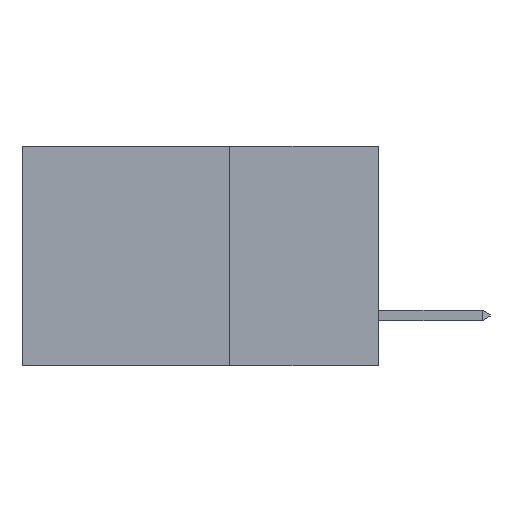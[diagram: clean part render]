
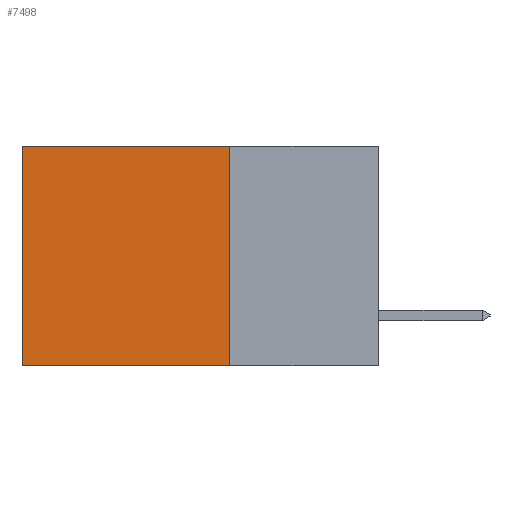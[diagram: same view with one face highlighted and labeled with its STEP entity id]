
A CAD part, left-side view. The second image highlights one B-rep face of the part: STEP entity #7498.
In plain terms, the highlighted planar face has unit normal (-1, 0, 0).
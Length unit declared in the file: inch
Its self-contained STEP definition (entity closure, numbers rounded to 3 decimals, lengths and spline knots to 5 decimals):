
#665 = VECTOR ( 'NONE', #9670, 39.37008 ) ;
#2373 = VERTEX_POINT ( 'NONE', #3122 ) ;
#2735 = VECTOR ( 'NONE', #9588, 39.37008 ) ;
#3122 = CARTESIAN_POINT ( 'NONE',  ( 0.2615, 0.6, 0. ) ) ;
#3633 = CARTESIAN_POINT ( 'NONE',  ( 0.2615, 0.6, -0.37 ) ) ;
#5329 = AXIS2_PLACEMENT_3D ( 'NONE', #10758, #12197, #13166 ) ;
#5588 = ORIENTED_EDGE ( 'NONE', *, *, #11758, .T. ) ;
#5737 = ORIENTED_EDGE ( 'NONE', *, *, #5966, .T. ) ;
#5966 = EDGE_CURVE ( 'NONE', #2373, #10109, #16597, .T. ) ;
#6397 = DIRECTION ( 'NONE',  ( 0., 0., -1. ) ) ;
#6584 = FACE_OUTER_BOUND ( 'NONE', #8172, .T. ) ;
#6719 = ORIENTED_EDGE ( 'NONE', *, *, #12212, .F. ) ;
#6962 = VECTOR ( 'NONE', #8562, 39.37008 ) ;
#7164 = CARTESIAN_POINT ( 'NONE',  ( 0.2615, 0.25, -0.37 ) ) ;
#7402 = LINE ( 'NONE', #7164, #6962 ) ;
#7498 = ADVANCED_FACE ( 'NONE', ( #6584 ), #14477, .F. ) ;
#8172 = EDGE_LOOP ( 'NONE', ( #5737, #11375, #6719, #5588 ) ) ;
#8562 = DIRECTION ( 'NONE',  ( 0., 1., 0. ) ) ;
#9190 = VERTEX_POINT ( 'NONE', #9952 ) ;
#9340 = VECTOR ( 'NONE', #6397, 39.37008 ) ;
#9588 = DIRECTION ( 'NONE',  ( 0., 1., 0. ) ) ;
#9670 = DIRECTION ( 'NONE',  ( 0., 0., -1. ) ) ;
#9754 = CARTESIAN_POINT ( 'NONE',  ( 0.2615, 0.6, -0.37 ) ) ;
#9952 = CARTESIAN_POINT ( 'NONE',  ( 0.2615, 0.25, -0.37 ) ) ;
#9980 = CARTESIAN_POINT ( 'NONE',  ( 0.2615, 0.25, 0. ) ) ;
#10109 = VERTEX_POINT ( 'NONE', #3633 ) ;
#10698 = LINE ( 'NONE', #13807, #2735 ) ;
#10758 = CARTESIAN_POINT ( 'NONE',  ( 0.2615, 0.25, -0.37 ) ) ;
#11246 = EDGE_CURVE ( 'NONE', #9190, #10109, #7402, .T. ) ;
#11375 = ORIENTED_EDGE ( 'NONE', *, *, #11246, .F. ) ;
#11758 = EDGE_CURVE ( 'NONE', #17719, #2373, #10698, .T. ) ;
#11944 = CARTESIAN_POINT ( 'NONE',  ( 0.2615, 0.25, -0.37 ) ) ;
#12197 = DIRECTION ( 'NONE',  ( 1., 0., 0. ) ) ;
#12212 = EDGE_CURVE ( 'NONE', #17719, #9190, #13113, .T. ) ;
#13113 = LINE ( 'NONE', #11944, #9340 ) ;
#13166 = DIRECTION ( 'NONE',  ( 0., 0., -1. ) ) ;
#13807 = CARTESIAN_POINT ( 'NONE',  ( 0.2615, 0.25, 0. ) ) ;
#14477 = PLANE ( 'NONE',  #5329 ) ;
#16597 = LINE ( 'NONE', #9754, #665 ) ;
#17719 = VERTEX_POINT ( 'NONE', #9980 ) ;
